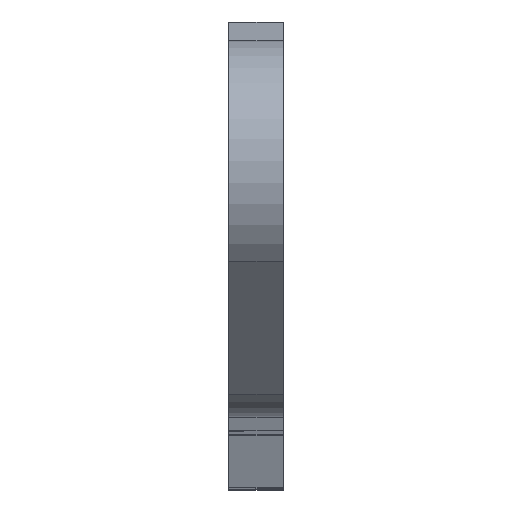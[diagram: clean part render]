
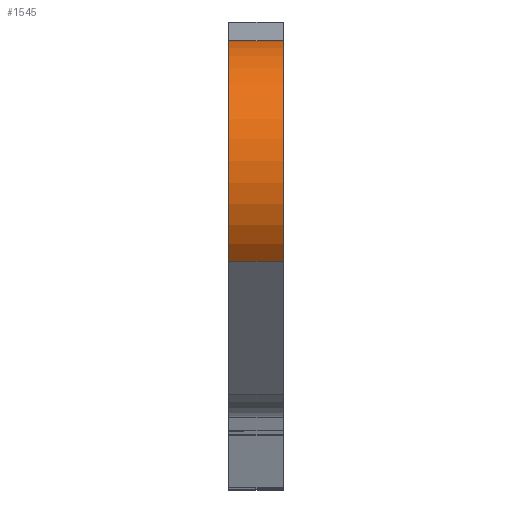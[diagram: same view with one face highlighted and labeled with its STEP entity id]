
A CAD part, top view. The second image highlights one B-rep face of the part: STEP entity #1545.
In plain terms, the highlighted cylindrical face has radius 5.563 mm (diameter 11.125 mm), a partial arc.
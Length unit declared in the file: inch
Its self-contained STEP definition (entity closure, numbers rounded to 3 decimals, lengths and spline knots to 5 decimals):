
#123=FACE_OUTER_BOUND('',#216,.T.);
#216=EDGE_LOOP('',(#1198,#1199,#1200,#1201));
#289=CIRCLE('',#1640,0.219);
#294=CIRCLE('',#1650,0.219);
#440=LINE('',#3579,#559);
#444=LINE('',#3588,#563);
#559=VECTOR('',#1860,0.3937);
#563=VECTOR('',#1870,0.3937);
#724=VERTEX_POINT('',#3556);
#725=VERTEX_POINT('',#3558);
#731=VERTEX_POINT('',#3576);
#734=VERTEX_POINT('',#3586);
#896=EDGE_CURVE('',#724,#725,#289,.T.);
#906=EDGE_CURVE('',#724,#731,#440,.T.);
#910=EDGE_CURVE('',#734,#731,#294,.T.);
#911=EDGE_CURVE('',#725,#734,#444,.T.);
#1198=ORIENTED_EDGE('',*,*,#910,.F.);
#1199=ORIENTED_EDGE('',*,*,#911,.F.);
#1200=ORIENTED_EDGE('',*,*,#896,.F.);
#1201=ORIENTED_EDGE('',*,*,#906,.T.);
#1493=CYLINDRICAL_SURFACE('',#1649,0.219);
#1545=ADVANCED_FACE('',(#123),#1493,.T.);
#1640=AXIS2_PLACEMENT_3D('',#3559,#1839,#1840);
#1649=AXIS2_PLACEMENT_3D('',#3585,#1866,#1867);
#1650=AXIS2_PLACEMENT_3D('',#3587,#1868,#1869);
#1839=DIRECTION('center_axis',(1.,0.,0.));
#1840=DIRECTION('ref_axis',(0.,1.,0.));
#1860=DIRECTION('',(-1.,0.,0.));
#1866=DIRECTION('center_axis',(-1.,0.,0.));
#1867=DIRECTION('ref_axis',(0.,1.,0.));
#1868=DIRECTION('center_axis',(-1.,0.,0.));
#1869=DIRECTION('ref_axis',(0.,1.,0.));
#1870=DIRECTION('',(-1.,0.,0.));
#3556=CARTESIAN_POINT('',(0.575,-0.031,3.26648));
#3558=CARTESIAN_POINT('',(0.575,-0.39606,3.42965));
#3559=CARTESIAN_POINT('Origin',(0.575,-0.25,3.26648));
#3576=CARTESIAN_POINT('',(0.485,-0.031,3.26648));
#3579=CARTESIAN_POINT('',(0.61543,-0.031,3.26648));
#3585=CARTESIAN_POINT('Origin',(0.61543,-0.25,3.26648));
#3586=CARTESIAN_POINT('',(0.485,-0.39606,3.42965));
#3587=CARTESIAN_POINT('Origin',(0.485,-0.25,3.26648));
#3588=CARTESIAN_POINT('',(0.61543,-0.39606,3.42965));
